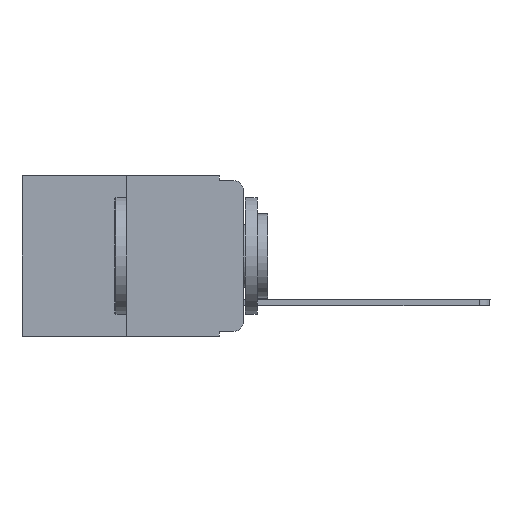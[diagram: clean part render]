
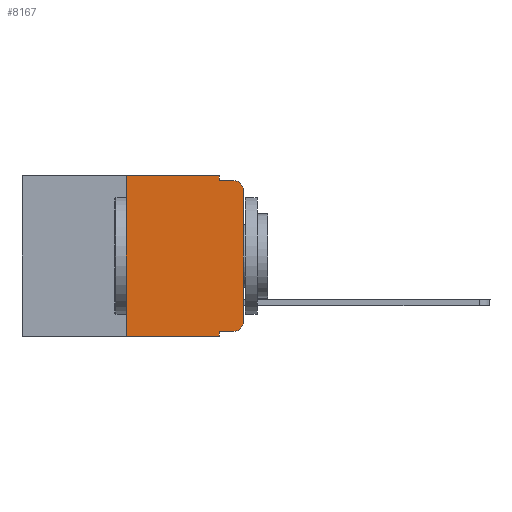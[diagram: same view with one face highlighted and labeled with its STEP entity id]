
A CAD part, left-side view. The second image highlights one B-rep face of the part: STEP entity #8167.
In plain terms, the highlighted planar face has unit normal (-1, 0, 0).
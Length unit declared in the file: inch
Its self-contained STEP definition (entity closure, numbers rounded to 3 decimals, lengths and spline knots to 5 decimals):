
#106 = VERTEX_POINT ( 'NONE', #1290 ) ;
#367 = VECTOR ( 'NONE', #5248, 39.37008 ) ;
#406 = DIRECTION ( 'NONE',  ( 0., -1., 0. ) ) ;
#650 = ORIENTED_EDGE ( 'NONE', *, *, #5943, .F. ) ;
#756 = CARTESIAN_POINT ( 'NONE',  ( 0., 0.473, 0. ) ) ;
#880 = EDGE_LOOP ( 'NONE', ( #14703, #2353, #650, #6247, #8614, #8750, #10563, #18044, #10644, #8019 ) ) ;
#1170 = VERTEX_POINT ( 'NONE', #12283 ) ;
#1179 = DIRECTION ( 'NONE',  ( 1., 0., 0. ) ) ;
#1287 = CARTESIAN_POINT ( 'NONE',  ( 0., 0.051, -0.333 ) ) ;
#1290 = CARTESIAN_POINT ( 'NONE',  ( 0., 0., -0.313 ) ) ;
#1433 = DIRECTION ( 'NONE',  ( -1., 0., 0. ) ) ;
#1642 = DIRECTION ( 'NONE',  ( 0., 0., -1. ) ) ;
#1669 = CARTESIAN_POINT ( 'NONE',  ( 0., 0.051, 0. ) ) ;
#1983 = EDGE_CURVE ( 'NONE', #16038, #12402, #2001, .T. ) ;
#2001 = LINE ( 'NONE', #8458, #2562 ) ;
#2353 = ORIENTED_EDGE ( 'NONE', *, *, #19399, .T. ) ;
#2417 = CARTESIAN_POINT ( 'NONE',  ( 0., 0.051, -0.01 ) ) ;
#2543 = VECTOR ( 'NONE', #19002, 39.37008 ) ;
#2562 = VECTOR ( 'NONE', #406, 39.37008 ) ;
#2577 = CIRCLE ( 'NONE', #3229, 0.02 ) ;
#2634 = AXIS2_PLACEMENT_3D ( 'NONE', #20885, #1433, #1642 ) ;
#2782 = CARTESIAN_POINT ( 'NONE',  ( 0., 0.02, -0.333 ) ) ;
#3229 = AXIS2_PLACEMENT_3D ( 'NONE', #18606, #20212, #20531 ) ;
#4014 = LINE ( 'NONE', #2417, #17295 ) ;
#4505 = EDGE_CURVE ( 'NONE', #8271, #7608, #5144, .T. ) ;
#4552 = LINE ( 'NONE', #7537, #16932 ) ;
#5060 = CARTESIAN_POINT ( 'NONE',  ( 0., 0.25, 0. ) ) ;
#5144 = LINE ( 'NONE', #1669, #367 ) ;
#5181 = CARTESIAN_POINT ( 'NONE',  ( 0., 0.051, 0. ) ) ;
#5248 = DIRECTION ( 'NONE',  ( 0., 0., -1. ) ) ;
#5484 = EDGE_CURVE ( 'NONE', #1170, #7608, #4552, .T. ) ;
#5664 = CARTESIAN_POINT ( 'NONE',  ( 0., 0., -0.03 ) ) ;
#5710 = DIRECTION ( 'NONE',  ( 0., -1., 0. ) ) ;
#5943 = EDGE_CURVE ( 'NONE', #8793, #19185, #4014, .T. ) ;
#6038 = CARTESIAN_POINT ( 'NONE',  ( 0., 0., 0. ) ) ;
#6142 = LINE ( 'NONE', #6038, #2543 ) ;
#6247 = ORIENTED_EDGE ( 'NONE', *, *, #18918, .F. ) ;
#6741 = DIRECTION ( 'NONE',  ( 0., 0., -1. ) ) ;
#6858 = CARTESIAN_POINT ( 'NONE',  ( 0., 0.25, 0. ) ) ;
#7537 = CARTESIAN_POINT ( 'NONE',  ( 0., 0.473, -0.343 ) ) ;
#7608 = VERTEX_POINT ( 'NONE', #11098 ) ;
#8019 = ORIENTED_EDGE ( 'NONE', *, *, #18353, .T. ) ;
#8167 = ADVANCED_FACE ( 'NONE', ( #12276 ), #16918, .F. ) ;
#8271 = VERTEX_POINT ( 'NONE', #1287 ) ;
#8458 = CARTESIAN_POINT ( 'NONE',  ( 0., 0.473, 0. ) ) ;
#8614 = ORIENTED_EDGE ( 'NONE', *, *, #1983, .F. ) ;
#8750 = ORIENTED_EDGE ( 'NONE', *, *, #10246, .F. ) ;
#8793 = VERTEX_POINT ( 'NONE', #14476 ) ;
#10015 = LINE ( 'NONE', #14448, #15096 ) ;
#10060 = CIRCLE ( 'NONE', #2634, 0.02 ) ;
#10246 = EDGE_CURVE ( 'NONE', #1170, #16038, #13499, .T. ) ;
#10563 = ORIENTED_EDGE ( 'NONE', *, *, #5484, .T. ) ;
#10644 = ORIENTED_EDGE ( 'NONE', *, *, #12487, .T. ) ;
#11013 = DIRECTION ( 'NONE',  ( 0., -1., 0. ) ) ;
#11098 = CARTESIAN_POINT ( 'NONE',  ( 0., 0.051, -0.343 ) ) ;
#12007 = VECTOR ( 'NONE', #17221, 39.37008 ) ;
#12276 = FACE_OUTER_BOUND ( 'NONE', #880, .T. ) ;
#12283 = CARTESIAN_POINT ( 'NONE',  ( 0., 0.25, -0.343 ) ) ;
#12402 = VERTEX_POINT ( 'NONE', #5181 ) ;
#12487 = EDGE_CURVE ( 'NONE', #8271, #13831, #15542, .T. ) ;
#13457 = VERTEX_POINT ( 'NONE', #5664 ) ;
#13499 = LINE ( 'NONE', #5060, #18736 ) ;
#13831 = VERTEX_POINT ( 'NONE', #2782 ) ;
#14448 = CARTESIAN_POINT ( 'NONE',  ( 0., 0.051, 0. ) ) ;
#14476 = CARTESIAN_POINT ( 'NONE',  ( 0., 0.051, -0.01 ) ) ;
#14703 = ORIENTED_EDGE ( 'NONE', *, *, #17051, .T. ) ;
#15096 = VECTOR ( 'NONE', #6741, 39.37008 ) ;
#15340 = DIRECTION ( 'NONE',  ( 0., 0., -1. ) ) ;
#15542 = LINE ( 'NONE', #15749, #12007 ) ;
#15749 = CARTESIAN_POINT ( 'NONE',  ( 0., 0.051, -0.333 ) ) ;
#15975 = AXIS2_PLACEMENT_3D ( 'NONE', #756, #1179, #15340 ) ;
#16038 = VERTEX_POINT ( 'NONE', #6858 ) ;
#16918 = PLANE ( 'NONE',  #15975 ) ;
#16932 = VECTOR ( 'NONE', #11013, 39.37008 ) ;
#17051 = EDGE_CURVE ( 'NONE', #106, #13457, #6142, .T. ) ;
#17221 = DIRECTION ( 'NONE',  ( 0., -1., 0. ) ) ;
#17295 = VECTOR ( 'NONE', #5710, 39.37008 ) ;
#18044 = ORIENTED_EDGE ( 'NONE', *, *, #4505, .F. ) ;
#18077 = CARTESIAN_POINT ( 'NONE',  ( 0., 0.02, -0.01 ) ) ;
#18353 = EDGE_CURVE ( 'NONE', #13831, #106, #2577, .T. ) ;
#18606 = CARTESIAN_POINT ( 'NONE',  ( 0., 0.02, -0.313 ) ) ;
#18736 = VECTOR ( 'NONE', #19624, 39.37008 ) ;
#18918 = EDGE_CURVE ( 'NONE', #12402, #8793, #10015, .T. ) ;
#19002 = DIRECTION ( 'NONE',  ( 0., 0., 1. ) ) ;
#19185 = VERTEX_POINT ( 'NONE', #18077 ) ;
#19399 = EDGE_CURVE ( 'NONE', #13457, #19185, #10060, .T. ) ;
#19624 = DIRECTION ( 'NONE',  ( 0., 0., 1. ) ) ;
#20212 = DIRECTION ( 'NONE',  ( -1., 0., 0. ) ) ;
#20531 = DIRECTION ( 'NONE',  ( 0., 0., -1. ) ) ;
#20885 = CARTESIAN_POINT ( 'NONE',  ( 0., 0.02, -0.03 ) ) ;
